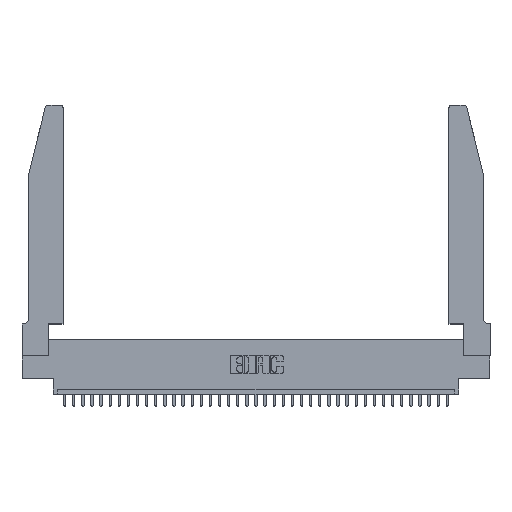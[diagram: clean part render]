
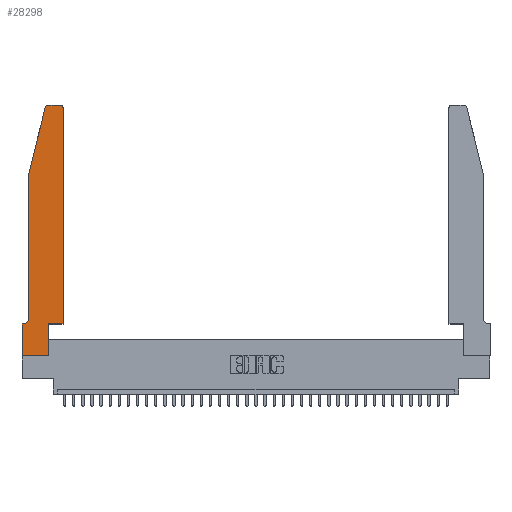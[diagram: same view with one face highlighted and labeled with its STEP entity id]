
A CAD part, top view. The second image highlights one B-rep face of the part: STEP entity #28298.
In plain terms, the highlighted planar face has unit normal (0, 0, 1).
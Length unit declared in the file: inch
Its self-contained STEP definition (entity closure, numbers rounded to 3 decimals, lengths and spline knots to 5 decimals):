
#253 = VERTEX_POINT ( 'NONE', #25023 ) ;
#731 = DIRECTION ( 'NONE',  ( 1., 0., 0. ) ) ;
#901 = VERTEX_POINT ( 'NONE', #17046 ) ;
#1242 = CIRCLE ( 'NONE', #19670, 0.07 ) ;
#1264 = LINE ( 'NONE', #9875, #30866 ) ;
#1581 = ORIENTED_EDGE ( 'NONE', *, *, #12657, .T. ) ;
#2324 = LINE ( 'NONE', #6593, #20269 ) ;
#2528 = ORIENTED_EDGE ( 'NONE', *, *, #6058, .T. ) ;
#2690 = FACE_OUTER_BOUND ( 'NONE', #19093, .T. ) ;
#3072 = CARTESIAN_POINT ( 'NONE',  ( 0.4205, 2.75, 0.37 ) ) ;
#3800 = VERTEX_POINT ( 'NONE', #20877 ) ;
#4214 = CARTESIAN_POINT ( 'NONE',  ( 0.4505, 0.35, 0.37 ) ) ;
#4388 = VERTEX_POINT ( 'NONE', #36314 ) ;
#4419 = ORIENTED_EDGE ( 'NONE', *, *, #29855, .T. ) ;
#4558 = VERTEX_POINT ( 'NONE', #3072 ) ;
#4562 = LINE ( 'NONE', #17606, #31068 ) ;
#5916 = DIRECTION ( 'NONE',  ( 1., 0., 0. ) ) ;
#6037 = EDGE_CURVE ( 'NONE', #4388, #24414, #27363, .T. ) ;
#6058 = EDGE_CURVE ( 'NONE', #10192, #4558, #28236, .T. ) ;
#6586 = VECTOR ( 'NONE', #28061, 39.37008 ) ;
#6593 = CARTESIAN_POINT ( 'NONE',  ( 0.0755, 2., 0.37 ) ) ;
#7999 = VERTEX_POINT ( 'NONE', #34969 ) ;
#8012 = ORIENTED_EDGE ( 'NONE', *, *, #18977, .T. ) ;
#8193 = DIRECTION ( 'NONE',  ( -1., 0., 0. ) ) ;
#9312 = DIRECTION ( 'NONE',  ( 0., 0., 1. ) ) ;
#9875 = CARTESIAN_POINT ( 'NONE',  ( 0.2605, 2.75, 0.37 ) ) ;
#10019 = CARTESIAN_POINT ( 'NONE',  ( 0., 0., 0.37 ) ) ;
#10179 = EDGE_CURVE ( 'NONE', #901, #253, #4562, .T. ) ;
#10192 = VERTEX_POINT ( 'NONE', #12318 ) ;
#10912 = EDGE_CURVE ( 'NONE', #14795, #901, #2324, .T. ) ;
#11545 = LINE ( 'NONE', #34040, #19260 ) ;
#11587 = DIRECTION ( 'NONE',  ( 0., 0., 1. ) ) ;
#12077 = ORIENTED_EDGE ( 'NONE', *, *, #23905, .T. ) ;
#12318 = CARTESIAN_POINT ( 'NONE',  ( 0.4505, 2.72, 0.37 ) ) ;
#12657 = EDGE_CURVE ( 'NONE', #36335, #14759, #14044, .T. ) ;
#14044 = LINE ( 'NONE', #21232, #36444 ) ;
#14358 = DIRECTION ( 'NONE',  ( 1., 0., 0. ) ) ;
#14759 = VERTEX_POINT ( 'NONE', #16742 ) ;
#14795 = VERTEX_POINT ( 'NONE', #36394 ) ;
#15155 = CARTESIAN_POINT ( 'NONE',  ( 0.284, 2.72, 0.37 ) ) ;
#16318 = DIRECTION ( 'NONE',  ( 0., -1., 0. ) ) ;
#16460 = LINE ( 'NONE', #36454, #22721 ) ;
#16742 = CARTESIAN_POINT ( 'NONE',  ( 0.2865, 0., 0.37 ) ) ;
#17046 = CARTESIAN_POINT ( 'NONE',  ( 0.0755, 2., 0.37 ) ) ;
#17111 = DIRECTION ( 'NONE',  ( 0., -1., 0. ) ) ;
#17170 = PLANE ( 'NONE',  #18472 ) ;
#17279 = DIRECTION ( 'NONE',  ( 0., 0., 1. ) ) ;
#17403 = CARTESIAN_POINT ( 'NONE',  ( 0.4205, 2.72, 0.37 ) ) ;
#17440 = LINE ( 'NONE', #33307, #6586 ) ;
#17606 = CARTESIAN_POINT ( 'NONE',  ( 0.0755, 2., 0.37 ) ) ;
#17837 = ORIENTED_EDGE ( 'NONE', *, *, #30036, .T. ) ;
#18125 = LINE ( 'NONE', #26719, #26150 ) ;
#18472 = AXIS2_PLACEMENT_3D ( 'NONE', #28401, #11587, #31550 ) ;
#18597 = DIRECTION ( 'NONE',  ( 0., 1., 0. ) ) ;
#18873 = DIRECTION ( 'NONE',  ( 1., 0., 0. ) ) ;
#18977 = EDGE_CURVE ( 'NONE', #3800, #14795, #21965, .T. ) ;
#19093 = EDGE_LOOP ( 'NONE', ( #12077, #8012, #21150, #32117, #17837, #4419, #36997, #1581, #34740, #32992, #29940, #2528 ) ) ;
#19260 = VECTOR ( 'NONE', #28049, 39.37008 ) ;
#19439 = EDGE_CURVE ( 'NONE', #14759, #4388, #11545, .T. ) ;
#19670 = AXIS2_PLACEMENT_3D ( 'NONE', #25580, #25457, #8193 ) ;
#20269 = VECTOR ( 'NONE', #26606, 39.37008 ) ;
#20877 = CARTESIAN_POINT ( 'NONE',  ( 0.284, 2.75, 0.37 ) ) ;
#21150 = ORIENTED_EDGE ( 'NONE', *, *, #10912, .T. ) ;
#21232 = CARTESIAN_POINT ( 'NONE',  ( 0., 0., 0.37 ) ) ;
#21965 = CIRCLE ( 'NONE', #35476, 0.03 ) ;
#22694 = AXIS2_PLACEMENT_3D ( 'NONE', #17403, #17279, #14358 ) ;
#22721 = VECTOR ( 'NONE', #16318, 39.37008 ) ;
#22802 = CARTESIAN_POINT ( 'NONE',  ( 0.4505, 0.35, 0.37 ) ) ;
#23762 = VERTEX_POINT ( 'NONE', #23963 ) ;
#23905 = EDGE_CURVE ( 'NONE', #4558, #3800, #1264, .T. ) ;
#23963 = CARTESIAN_POINT ( 'NONE',  ( 0.0055, 0.35, 0.37 ) ) ;
#24414 = VERTEX_POINT ( 'NONE', #4214 ) ;
#24915 = EDGE_CURVE ( 'NONE', #7999, #36335, #16460, .T. ) ;
#25023 = CARTESIAN_POINT ( 'NONE',  ( 0.0755, 0.42, 0.37 ) ) ;
#25457 = DIRECTION ( 'NONE',  ( 0., 0., -1. ) ) ;
#25580 = CARTESIAN_POINT ( 'NONE',  ( 0.0055, 0.42, 0.37 ) ) ;
#25618 = DIRECTION ( 'NONE',  ( -1., 0., 0. ) ) ;
#26150 = VECTOR ( 'NONE', #18597, 39.37008 ) ;
#26410 = EDGE_CURVE ( 'NONE', #24414, #10192, #18125, .T. ) ;
#26606 = DIRECTION ( 'NONE',  ( -0.239, -0.971, 0. ) ) ;
#26719 = CARTESIAN_POINT ( 'NONE',  ( 0.4505, 0.35, 0.37 ) ) ;
#27363 = LINE ( 'NONE', #22802, #28656 ) ;
#28049 = DIRECTION ( 'NONE',  ( 0., 1., 0. ) ) ;
#28061 = DIRECTION ( 'NONE',  ( -1., 0., 0. ) ) ;
#28236 = CIRCLE ( 'NONE', #22694, 0.03 ) ;
#28298 = ADVANCED_FACE ( 'NONE', ( #2690 ), #17170, .T. ) ;
#28401 = CARTESIAN_POINT ( 'NONE',  ( 0., 0.35, 0.37 ) ) ;
#28656 = VECTOR ( 'NONE', #5916, 39.37008 ) ;
#29855 = EDGE_CURVE ( 'NONE', #23762, #7999, #17440, .T. ) ;
#29940 = ORIENTED_EDGE ( 'NONE', *, *, #26410, .T. ) ;
#30036 = EDGE_CURVE ( 'NONE', #253, #23762, #1242, .T. ) ;
#30866 = VECTOR ( 'NONE', #25618, 39.37008 ) ;
#31068 = VECTOR ( 'NONE', #17111, 39.37008 ) ;
#31550 = DIRECTION ( 'NONE',  ( 1., 0., 0. ) ) ;
#32117 = ORIENTED_EDGE ( 'NONE', *, *, #10179, .T. ) ;
#32992 = ORIENTED_EDGE ( 'NONE', *, *, #6037, .T. ) ;
#33307 = CARTESIAN_POINT ( 'NONE',  ( 0.0755, 0.35, 0.37 ) ) ;
#34040 = CARTESIAN_POINT ( 'NONE',  ( 0.2865, 0.35, 0.37 ) ) ;
#34740 = ORIENTED_EDGE ( 'NONE', *, *, #19439, .T. ) ;
#34969 = CARTESIAN_POINT ( 'NONE',  ( 0., 0.35, 0.37 ) ) ;
#35476 = AXIS2_PLACEMENT_3D ( 'NONE', #15155, #9312, #731 ) ;
#36314 = CARTESIAN_POINT ( 'NONE',  ( 0.2865, 0.35, 0.37 ) ) ;
#36335 = VERTEX_POINT ( 'NONE', #10019 ) ;
#36394 = CARTESIAN_POINT ( 'NONE',  ( 0.25487, 2.72718, 0.37 ) ) ;
#36444 = VECTOR ( 'NONE', #18873, 39.37008 ) ;
#36454 = CARTESIAN_POINT ( 'NONE',  ( 0., 0., 0.37 ) ) ;
#36997 = ORIENTED_EDGE ( 'NONE', *, *, #24915, .T. ) ;
